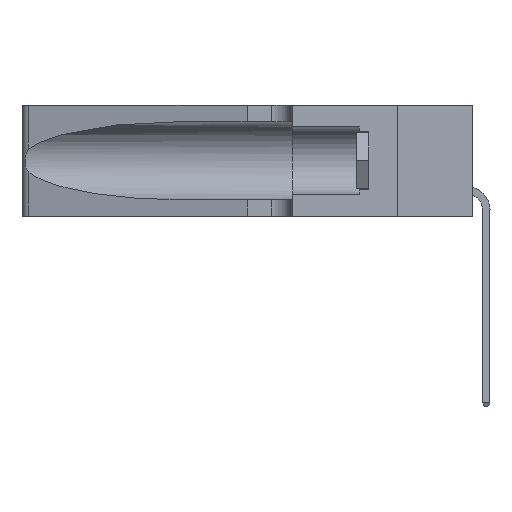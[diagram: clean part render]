
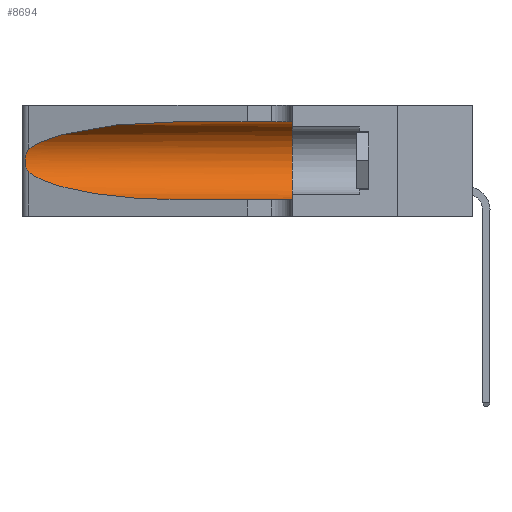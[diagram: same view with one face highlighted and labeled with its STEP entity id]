
A CAD part, left-side view. The second image highlights one B-rep face of the part: STEP entity #8694.
In plain terms, the highlighted cylindrical face has radius 3.308 mm (diameter 6.617 mm), a partial arc.
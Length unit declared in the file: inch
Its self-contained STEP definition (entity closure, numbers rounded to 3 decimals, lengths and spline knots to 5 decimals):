
#96 = FACE_OUTER_BOUND ( 'NONE', #8781, .T. ) ;
#876 = ORIENTED_EDGE ( 'NONE', *, *, #3104, .T. ) ;
#1205 = CARTESIAN_POINT ( 'NONE',  ( 0.18966, 0.96281, 0.05475 ) ) ;
#1247 = EDGE_CURVE ( 'NONE', #10938, #10239, #2802, .T. ) ;
#1304 = VECTOR ( 'NONE', #9584, 39.37008 ) ;
#1389 = CARTESIAN_POINT ( 'NONE',  ( 0.25487, 1.22718, 0.22369 ) ) ;
#1515 = LINE ( 'NONE', #16048, #1304 ) ;
#1870 = CARTESIAN_POINT ( 'NONE',  ( 0.1305, 1.61858, 0.185 ) ) ;
#1888 = CARTESIAN_POINT ( 'NONE',  ( 0.25854, 1.2359, 0.20912 ) ) ;
#2042 = AXIS2_PLACEMENT_3D ( 'NONE', #11345, #9947, #7341 ) ;
#2385 = VERTEX_POINT ( 'NONE', #16426 ) ;
#2802 =( BOUNDED_CURVE ( )  B_SPLINE_CURVE ( 3, ( #10720, #4046, #2819, #1389 ),
 .UNSPECIFIED., .F., .F. ) 
 B_SPLINE_CURVE_WITH_KNOTS ( ( 4, 4 ),
 ( 1.5708, 2.84003 ),
 .UNSPECIFIED. ) 
 CURVE ( )  GEOMETRIC_REPRESENTATION_ITEM ( )  RATIONAL_B_SPLINE_CURVE ( ( 1., 0.87, 0.87, 1. ) ) 
 REPRESENTATION_ITEM ( '' )  );
#2819 = CARTESIAN_POINT ( 'NONE',  ( 0.2373, 1.15595, 0.28018 ) ) ;
#2875 = ORIENTED_EDGE ( 'NONE', *, *, #13303, .T. ) ;
#3104 = EDGE_CURVE ( 'NONE', #15263, #15323, #16635, .T. ) ;
#3879 = EDGE_CURVE ( 'NONE', #11572, #2385, #9811, .T. ) ;
#3918 = CARTESIAN_POINT ( 'NONE',  ( 0.1305, 0.72297, 0.05475 ) ) ;
#4046 = CARTESIAN_POINT ( 'NONE',  ( 0.18966, 0.96281, 0.31525 ) ) ;
#4790 = ORIENTED_EDGE ( 'NONE', *, *, #1247, .T. ) ;
#4832 = CARTESIAN_POINT ( 'NONE',  ( 0.25487, 1.22718, 0.14631 ) ) ;
#4995 = CARTESIAN_POINT ( 'NONE',  ( 0.1305, 0.72297, 0.05475 ) ) ;
#5234 = CARTESIAN_POINT ( 'NONE',  ( 0.25487, 1.22718, 0.14631 ) ) ;
#5320 = CARTESIAN_POINT ( 'NONE',  ( 0.26017, 1.23833, 0.17102 ) ) ;
#5831 = VECTOR ( 'NONE', #9009, 39.37008 ) ;
#5934 = DIRECTION ( 'NONE',  ( 0., 0., -1. ) ) ;
#6208 = CARTESIAN_POINT ( 'NONE',  ( 0.25487, 1.22718, 0.22369 ) ) ;
#6652 = CARTESIAN_POINT ( 'NONE',  ( 0.26075, 1.23896, 0.178 ) ) ;
#7136 = DIRECTION ( 'NONE',  ( 0., -1., 0. ) ) ;
#7341 = DIRECTION ( 'NONE',  ( 0., 0., 1. ) ) ;
#7663 = CARTESIAN_POINT ( 'NONE',  ( 0.1305, 0.35, 0.31525 ) ) ;
#7956 = CARTESIAN_POINT ( 'NONE',  ( 0.25639, 1.23186, 0.15144 ) ) ;
#8694 = ADVANCED_FACE ( 'NONE', ( #96 ), #11019, .F. ) ;
#8781 = EDGE_LOOP ( 'NONE', ( #4790, #2875, #876, #11908, #14077, #10652 ) ) ;
#9009 = DIRECTION ( 'NONE',  ( 0., -1., 0. ) ) ;
#9292 = CARTESIAN_POINT ( 'NONE',  ( 0.25555, 1.22993, 0.14849 ) ) ;
#9309 = LINE ( 'NONE', #10253, #5831 ) ;
#9584 = DIRECTION ( 'NONE',  ( 0., -1., 0. ) ) ;
#9762 = CARTESIAN_POINT ( 'NONE',  ( 0.25639, 1.23184, 0.21858 ) ) ;
#9811 = CIRCLE ( 'NONE', #2042, 0.13025 ) ;
#9947 = DIRECTION ( 'NONE',  ( 0., 1., 0. ) ) ;
#10239 = VERTEX_POINT ( 'NONE', #6208 ) ;
#10253 = CARTESIAN_POINT ( 'NONE',  ( 0.1305, 1.61858, 0.31525 ) ) ;
#10652 = ORIENTED_EDGE ( 'NONE', *, *, #14722, .F. ) ;
#10720 = CARTESIAN_POINT ( 'NONE',  ( 0.1305, 0.72297, 0.31525 ) ) ;
#10930 = CARTESIAN_POINT ( 'NONE',  ( 0.25487, 1.22718, 0.22369 ) ) ;
#10938 = VERTEX_POINT ( 'NONE', #12487 ) ;
#11019 = CYLINDRICAL_SURFACE ( 'NONE', #16793, 0.13025 ) ;
#11345 = CARTESIAN_POINT ( 'NONE',  ( 0.1305, 0.35, 0.185 ) ) ;
#11572 = VERTEX_POINT ( 'NONE', #7663 ) ;
#11908 = ORIENTED_EDGE ( 'NONE', *, *, #12819, .T. ) ;
#11927 = CARTESIAN_POINT ( 'NONE',  ( 0.26075, 1.23896, 0.19203 ) ) ;
#11990 = CARTESIAN_POINT ( 'NONE',  ( 0.25787, 1.23484, 0.2124 ) ) ;
#12487 = CARTESIAN_POINT ( 'NONE',  ( 0.1305, 0.72297, 0.31525 ) ) ;
#12819 = EDGE_CURVE ( 'NONE', #15323, #2385, #1515, .T. ) ;
#13303 = EDGE_CURVE ( 'NONE', #10239, #15263, #16110, .T. ) ;
#14077 = ORIENTED_EDGE ( 'NONE', *, *, #3879, .F. ) ;
#14556 = CARTESIAN_POINT ( 'NONE',  ( 0.25856, 1.23593, 0.16098 ) ) ;
#14722 = EDGE_CURVE ( 'NONE', #10938, #11572, #9309, .T. ) ;
#15021 = CARTESIAN_POINT ( 'NONE',  ( 0.25555, 1.22994, 0.2215 ) ) ;
#15263 = VERTEX_POINT ( 'NONE', #4832 ) ;
#15323 = VERTEX_POINT ( 'NONE', #4995 ) ;
#15669 = CARTESIAN_POINT ( 'NONE',  ( 0.2373, 1.15595, 0.08982 ) ) ;
#15866 = CARTESIAN_POINT ( 'NONE',  ( 0.25789, 1.23486, 0.15765 ) ) ;
#15927 = CARTESIAN_POINT ( 'NONE',  ( 0.25487, 1.22718, 0.14631 ) ) ;
#16048 = CARTESIAN_POINT ( 'NONE',  ( 0.1305, 1.61858, 0.05475 ) ) ;
#16110 = B_SPLINE_CURVE_WITH_KNOTS ( 'NONE', 3,
 ( #10930, #15021, #9762, #11990, #1888, #17160, #11927, #6652, #5320, #14556, #15866, #7956, #9292, #15927 ),
 .UNSPECIFIED., .F., .F.,
 ( 4, 2, 2, 2, 2, 2, 4 ),
 ( 0., 0.00027, 0.00053, 0.00107, 0.0016, 0.00187, 0.00214 ),
 .UNSPECIFIED. ) ;
#16426 = CARTESIAN_POINT ( 'NONE',  ( 0.1305, 0.35, 0.05475 ) ) ;
#16635 =( BOUNDED_CURVE ( )  B_SPLINE_CURVE ( 3, ( #5234, #15669, #1205, #3918 ),
 .UNSPECIFIED., .F., .F. ) 
 B_SPLINE_CURVE_WITH_KNOTS ( ( 4, 4 ),
 ( 3.44316, 4.71239 ),
 .UNSPECIFIED. ) 
 CURVE ( )  GEOMETRIC_REPRESENTATION_ITEM ( )  RATIONAL_B_SPLINE_CURVE ( ( 1., 0.87, 0.87, 1. ) ) 
 REPRESENTATION_ITEM ( '' )  );
#16793 = AXIS2_PLACEMENT_3D ( 'NONE', #1870, #7136, #5934 ) ;
#17160 = CARTESIAN_POINT ( 'NONE',  ( 0.26018, 1.23835, 0.19895 ) ) ;
